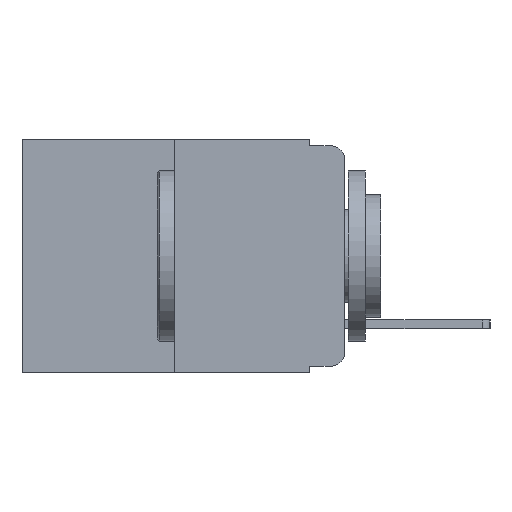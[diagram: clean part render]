
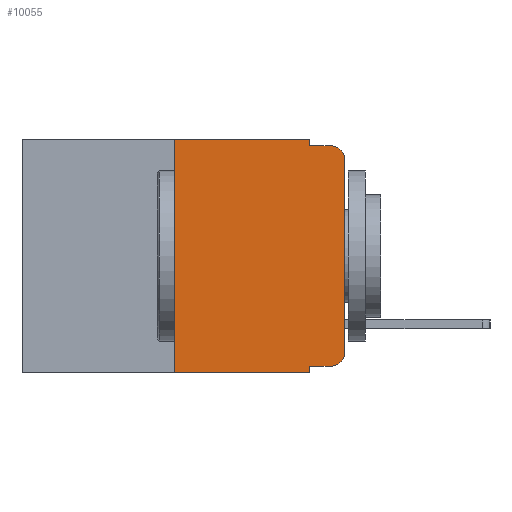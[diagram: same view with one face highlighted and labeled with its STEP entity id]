
A CAD part, left-side view. The second image highlights one B-rep face of the part: STEP entity #10055.
In plain terms, the highlighted planar face has unit normal (-1, 0, 0).
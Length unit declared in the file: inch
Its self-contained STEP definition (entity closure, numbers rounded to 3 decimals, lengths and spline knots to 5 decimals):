
#89 = DIRECTION ( 'NONE',  ( 0., -1., 0. ) ) ;
#525 = CARTESIAN_POINT ( 'NONE',  ( 0., 0., 0. ) ) ;
#542 = LINE ( 'NONE', #14079, #6948 ) ;
#590 = CARTESIAN_POINT ( 'NONE',  ( 0., 0.02, -0.03 ) ) ;
#669 = CARTESIAN_POINT ( 'NONE',  ( 0., 0.25, 0. ) ) ;
#980 = AXIS2_PLACEMENT_3D ( 'NONE', #2650, #13386, #13671 ) ;
#1711 = LINE ( 'NONE', #16055, #8091 ) ;
#1838 = VERTEX_POINT ( 'NONE', #2745 ) ;
#1960 = DIRECTION ( 'NONE',  ( 0., 0., -1. ) ) ;
#2337 = ORIENTED_EDGE ( 'NONE', *, *, #7556, .F. ) ;
#2444 = EDGE_CURVE ( 'NONE', #14835, #10330, #14667, .T. ) ;
#2650 = CARTESIAN_POINT ( 'NONE',  ( 0., 0.02, -0.313 ) ) ;
#2677 = DIRECTION ( 'NONE',  ( 1., 0., 0. ) ) ;
#2745 = CARTESIAN_POINT ( 'NONE',  ( 0., 0., -0.03 ) ) ;
#3030 = LINE ( 'NONE', #6230, #12776 ) ;
#3254 = CARTESIAN_POINT ( 'NONE',  ( 0., 0.051, -0.343 ) ) ;
#3899 = DIRECTION ( 'NONE',  ( 0., 0., -1. ) ) ;
#3922 = ORIENTED_EDGE ( 'NONE', *, *, #2444, .T. ) ;
#3949 = CARTESIAN_POINT ( 'NONE',  ( 0., 0.02, -0.01 ) ) ;
#4140 = EDGE_CURVE ( 'NONE', #5777, #14835, #3030, .T. ) ;
#4356 = EDGE_CURVE ( 'NONE', #13425, #5798, #542, .T. ) ;
#4574 = CARTESIAN_POINT ( 'NONE',  ( 0., 0.051, -0.01 ) ) ;
#4695 = CIRCLE ( 'NONE', #9611, 0.02 ) ;
#4989 = EDGE_CURVE ( 'NONE', #5777, #5798, #12947, .T. ) ;
#5777 = VERTEX_POINT ( 'NONE', #13315 ) ;
#5798 = VERTEX_POINT ( 'NONE', #3254 ) ;
#5829 = EDGE_CURVE ( 'NONE', #13425, #15786, #15849, .T. ) ;
#6088 = ORIENTED_EDGE ( 'NONE', *, *, #5829, .F. ) ;
#6230 = CARTESIAN_POINT ( 'NONE',  ( 0., 0.051, -0.333 ) ) ;
#6622 = FACE_OUTER_BOUND ( 'NONE', #14102, .T. ) ;
#6810 = VECTOR ( 'NONE', #9592, 39.37008 ) ;
#6948 = VECTOR ( 'NONE', #89, 39.37008 ) ;
#7275 = CARTESIAN_POINT ( 'NONE',  ( 0., 0.25, 0. ) ) ;
#7556 = EDGE_CURVE ( 'NONE', #15225, #15679, #9387, .T. ) ;
#7617 = AXIS2_PLACEMENT_3D ( 'NONE', #10396, #2677, #11626 ) ;
#7905 = ORIENTED_EDGE ( 'NONE', *, *, #10222, .T. ) ;
#8091 = VECTOR ( 'NONE', #8779, 39.37008 ) ;
#8452 = EDGE_CURVE ( 'NONE', #15679, #14657, #8922, .T. ) ;
#8474 = EDGE_CURVE ( 'NONE', #15786, #15225, #1711, .T. ) ;
#8655 = CARTESIAN_POINT ( 'NONE',  ( 0., 0.051, -0.01 ) ) ;
#8779 = DIRECTION ( 'NONE',  ( 0., -1., 0. ) ) ;
#8922 = LINE ( 'NONE', #8655, #12296 ) ;
#8975 = VECTOR ( 'NONE', #11975, 39.37008 ) ;
#9327 = EDGE_CURVE ( 'NONE', #1838, #14657, #4695, .T. ) ;
#9387 = LINE ( 'NONE', #15464, #8975 ) ;
#9422 = VECTOR ( 'NONE', #10988, 39.37008 ) ;
#9592 = DIRECTION ( 'NONE',  ( 0., 0., 1. ) ) ;
#9611 = AXIS2_PLACEMENT_3D ( 'NONE', #590, #9651, #1960 ) ;
#9651 = DIRECTION ( 'NONE',  ( -1., 0., 0. ) ) ;
#9869 = CARTESIAN_POINT ( 'NONE',  ( 0., 0., -0.313 ) ) ;
#9919 = DIRECTION ( 'NONE',  ( 0., -1., 0. ) ) ;
#9925 = LINE ( 'NONE', #525, #6810 ) ;
#9984 = ORIENTED_EDGE ( 'NONE', *, *, #4989, .F. ) ;
#10055 = ADVANCED_FACE ( 'NONE', ( #6622 ), #11575, .F. ) ;
#10222 = EDGE_CURVE ( 'NONE', #10330, #1838, #9925, .T. ) ;
#10330 = VERTEX_POINT ( 'NONE', #9869 ) ;
#10396 = CARTESIAN_POINT ( 'NONE',  ( 0., 0.473, 0. ) ) ;
#10988 = DIRECTION ( 'NONE',  ( 0., 0., 1. ) ) ;
#11334 = ORIENTED_EDGE ( 'NONE', *, *, #9327, .T. ) ;
#11575 = PLANE ( 'NONE',  #7617 ) ;
#11626 = DIRECTION ( 'NONE',  ( 0., 0., -1. ) ) ;
#11734 = ORIENTED_EDGE ( 'NONE', *, *, #8452, .F. ) ;
#11975 = DIRECTION ( 'NONE',  ( 0., 0., -1. ) ) ;
#12296 = VECTOR ( 'NONE', #9919, 39.37008 ) ;
#12505 = ORIENTED_EDGE ( 'NONE', *, *, #8474, .F. ) ;
#12582 = VECTOR ( 'NONE', #3899, 39.37008 ) ;
#12776 = VECTOR ( 'NONE', #13785, 39.37008 ) ;
#12872 = ORIENTED_EDGE ( 'NONE', *, *, #4356, .T. ) ;
#12947 = LINE ( 'NONE', #13919, #12582 ) ;
#13103 = CARTESIAN_POINT ( 'NONE',  ( 0., 0.02, -0.333 ) ) ;
#13241 = ORIENTED_EDGE ( 'NONE', *, *, #4140, .T. ) ;
#13315 = CARTESIAN_POINT ( 'NONE',  ( 0., 0.051, -0.333 ) ) ;
#13386 = DIRECTION ( 'NONE',  ( -1., 0., 0. ) ) ;
#13425 = VERTEX_POINT ( 'NONE', #15619 ) ;
#13671 = DIRECTION ( 'NONE',  ( 0., 0., -1. ) ) ;
#13785 = DIRECTION ( 'NONE',  ( 0., -1., 0. ) ) ;
#13849 = CARTESIAN_POINT ( 'NONE',  ( 0., 0.051, 0. ) ) ;
#13919 = CARTESIAN_POINT ( 'NONE',  ( 0., 0.051, 0. ) ) ;
#14079 = CARTESIAN_POINT ( 'NONE',  ( 0., 0.473, -0.343 ) ) ;
#14102 = EDGE_LOOP ( 'NONE', ( #7905, #11334, #11734, #2337, #12505, #6088, #12872, #9984, #13241, #3922 ) ) ;
#14657 = VERTEX_POINT ( 'NONE', #3949 ) ;
#14667 = CIRCLE ( 'NONE', #980, 0.02 ) ;
#14835 = VERTEX_POINT ( 'NONE', #13103 ) ;
#15225 = VERTEX_POINT ( 'NONE', #13849 ) ;
#15464 = CARTESIAN_POINT ( 'NONE',  ( 0., 0.051, 0. ) ) ;
#15619 = CARTESIAN_POINT ( 'NONE',  ( 0., 0.25, -0.343 ) ) ;
#15679 = VERTEX_POINT ( 'NONE', #4574 ) ;
#15786 = VERTEX_POINT ( 'NONE', #7275 ) ;
#15849 = LINE ( 'NONE', #669, #9422 ) ;
#16055 = CARTESIAN_POINT ( 'NONE',  ( 0., 0.473, 0. ) ) ;
